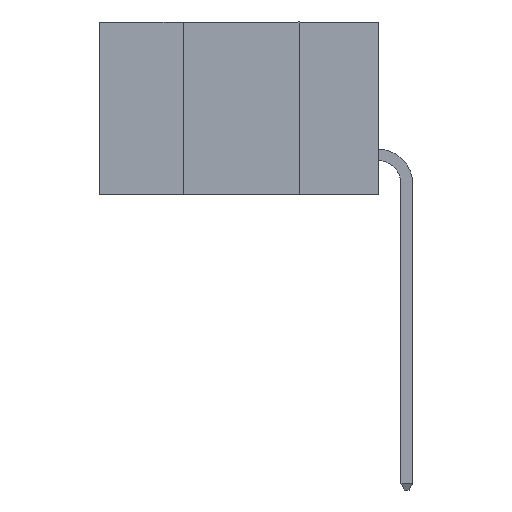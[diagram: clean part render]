
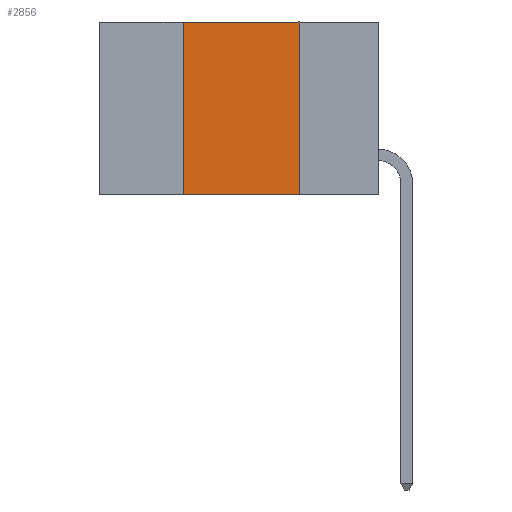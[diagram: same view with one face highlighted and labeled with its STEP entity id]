
A CAD part, left-side view. The second image highlights one B-rep face of the part: STEP entity #2856.
In plain terms, the highlighted planar face has unit normal (-1, 0, 0).
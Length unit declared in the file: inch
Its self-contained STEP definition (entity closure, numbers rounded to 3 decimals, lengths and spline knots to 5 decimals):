
#217 = EDGE_CURVE ( 'NONE', #11097, #13951, #8578, .T. ) ;
#506 = CARTESIAN_POINT ( 'NONE',  ( 0., 0.42, -0.37 ) ) ;
#1336 = DIRECTION ( 'NONE',  ( 0., -1., 0. ) ) ;
#1577 = DIRECTION ( 'NONE',  ( 0., 0., -1. ) ) ;
#2029 = ORIENTED_EDGE ( 'NONE', *, *, #15822, .F. ) ;
#2856 = ADVANCED_FACE ( 'NONE', ( #9774 ), #13605, .F. ) ;
#2981 = CARTESIAN_POINT ( 'NONE',  ( 0., 0.6, -0.37 ) ) ;
#3552 = VERTEX_POINT ( 'NONE', #5250 ) ;
#3581 = EDGE_CURVE ( 'NONE', #11097, #5731, #17757, .T. ) ;
#4192 = EDGE_LOOP ( 'NONE', ( #2029, #12733, #14648, #16935 ) ) ;
#4455 = LINE ( 'NONE', #17385, #7761 ) ;
#4489 = VECTOR ( 'NONE', #1577, 39.37008 ) ;
#4743 = CARTESIAN_POINT ( 'NONE',  ( 0., 0.42, -0.37 ) ) ;
#4822 = DIRECTION ( 'NONE',  ( 0., 0., 1. ) ) ;
#5250 = CARTESIAN_POINT ( 'NONE',  ( 0., 0.17, 0. ) ) ;
#5731 = VERTEX_POINT ( 'NONE', #14904 ) ;
#5947 = CARTESIAN_POINT ( 'NONE',  ( 0., 0.17, -0.37 ) ) ;
#7761 = VECTOR ( 'NONE', #16605, 39.37008 ) ;
#8137 = VECTOR ( 'NONE', #1336, 39.37008 ) ;
#8578 = LINE ( 'NONE', #2981, #8137 ) ;
#8756 = AXIS2_PLACEMENT_3D ( 'NONE', #13240, #13182, #12965 ) ;
#9774 = FACE_OUTER_BOUND ( 'NONE', #4192, .T. ) ;
#11097 = VERTEX_POINT ( 'NONE', #506 ) ;
#11480 = LINE ( 'NONE', #5947, #4489 ) ;
#12733 = ORIENTED_EDGE ( 'NONE', *, *, #13086, .F. ) ;
#12965 = DIRECTION ( 'NONE',  ( 0., 0., -1. ) ) ;
#13086 = EDGE_CURVE ( 'NONE', #5731, #3552, #4455, .T. ) ;
#13182 = DIRECTION ( 'NONE',  ( 1., 0., 0. ) ) ;
#13240 = CARTESIAN_POINT ( 'NONE',  ( 0., 0.6, 0. ) ) ;
#13605 = PLANE ( 'NONE',  #8756 ) ;
#13951 = VERTEX_POINT ( 'NONE', #14779 ) ;
#14235 = VECTOR ( 'NONE', #4822, 39.37008 ) ;
#14648 = ORIENTED_EDGE ( 'NONE', *, *, #3581, .F. ) ;
#14779 = CARTESIAN_POINT ( 'NONE',  ( 0., 0.17, -0.37 ) ) ;
#14904 = CARTESIAN_POINT ( 'NONE',  ( 0., 0.42, 0. ) ) ;
#15822 = EDGE_CURVE ( 'NONE', #3552, #13951, #11480, .T. ) ;
#16605 = DIRECTION ( 'NONE',  ( 0., -1., 0. ) ) ;
#16935 = ORIENTED_EDGE ( 'NONE', *, *, #217, .T. ) ;
#17385 = CARTESIAN_POINT ( 'NONE',  ( 0., 0.6, 0. ) ) ;
#17757 = LINE ( 'NONE', #4743, #14235 ) ;
